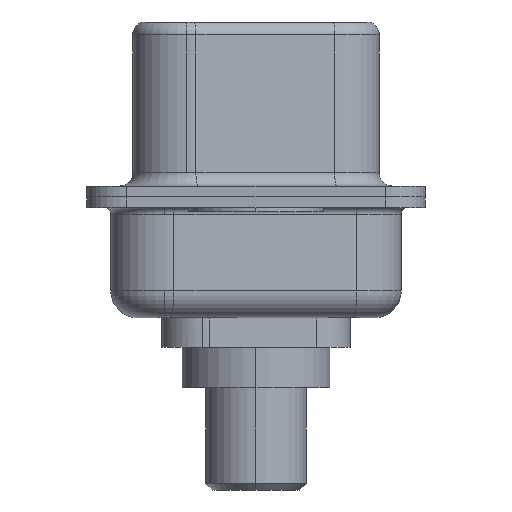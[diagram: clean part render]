
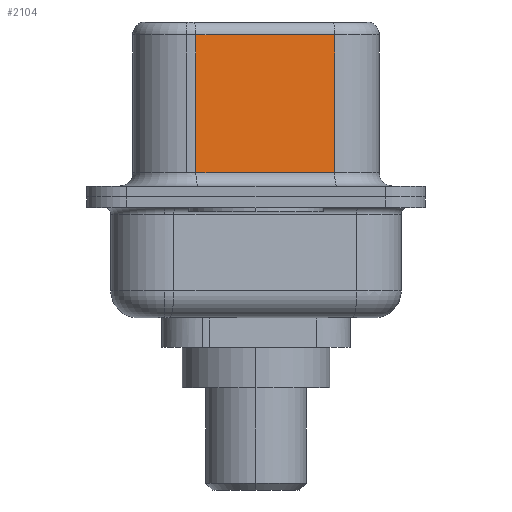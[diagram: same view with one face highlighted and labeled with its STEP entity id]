
A CAD part, left-side view. The second image highlights one B-rep face of the part: STEP entity #2104.
In plain terms, the highlighted planar face has unit normal (-0.985, -0.174, 0).
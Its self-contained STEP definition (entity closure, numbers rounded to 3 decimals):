
#248 = PLANE ( 'NONE',  #9617 ) ;
#559 = VECTOR ( 'NONE', #8483, 1000. ) ;
#745 = ORIENTED_EDGE ( 'NONE', *, *, #12222, .T. ) ;
#1006 = DIRECTION ( 'NONE',  ( -0.174, 0.985, 0. ) ) ;
#1617 = LINE ( 'NONE', #11188, #9682 ) ;
#2104 = ADVANCED_FACE ( 'NONE', ( #5008 ), #248, .F. ) ;
#2710 = VERTEX_POINT ( 'NONE', #4059 ) ;
#2716 = VECTOR ( 'NONE', #4438, 1000. ) ;
#3875 = LINE ( 'NONE', #8661, #12295 ) ;
#4059 = CARTESIAN_POINT ( 'NONE',  ( 4.565, -2.927, 0.9 ) ) ;
#4246 = EDGE_CURVE ( 'NONE', #11833, #2710, #3875, .T. ) ;
#4438 = DIRECTION ( 'NONE',  ( 0.174, -0.985, 0. ) ) ;
#4472 = CARTESIAN_POINT ( 'NONE',  ( 4.565, -2.927, 0.9 ) ) ;
#5008 = FACE_OUTER_BOUND ( 'NONE', #8089, .T. ) ;
#5394 = LINE ( 'NONE', #4472, #2716 ) ;
#6301 = ORIENTED_EDGE ( 'NONE', *, *, #11451, .T. ) ;
#6563 = CARTESIAN_POINT ( 'NONE',  ( 4.565, -2.927, 6.02 ) ) ;
#6676 = DIRECTION ( 'NONE',  ( 0.985, 0.174, 0. ) ) ;
#7121 = EDGE_CURVE ( 'NONE', #9130, #2710, #5394, .T. ) ;
#7491 = CARTESIAN_POINT ( 'NONE',  ( 3.655, 2.233, 6.02 ) ) ;
#8089 = EDGE_LOOP ( 'NONE', ( #8519, #745, #6301, #8365 ) ) ;
#8131 = DIRECTION ( 'NONE',  ( 0., 0., -1. ) ) ;
#8365 = ORIENTED_EDGE ( 'NONE', *, *, #7121, .T. ) ;
#8483 = DIRECTION ( 'NONE',  ( -0.174, 0.985, 0. ) ) ;
#8519 = ORIENTED_EDGE ( 'NONE', *, *, #4246, .F. ) ;
#8661 = CARTESIAN_POINT ( 'NONE',  ( 4.565, -2.927, 6.52 ) ) ;
#9130 = VERTEX_POINT ( 'NONE', #13201 ) ;
#9617 = AXIS2_PLACEMENT_3D ( 'NONE', #13203, #6676, #1006 ) ;
#9682 = VECTOR ( 'NONE', #8131, 1000. ) ;
#10248 = DIRECTION ( 'NONE',  ( 0., 0., -1. ) ) ;
#11133 = LINE ( 'NONE', #13647, #559 ) ;
#11170 = VERTEX_POINT ( 'NONE', #7491 ) ;
#11188 = CARTESIAN_POINT ( 'NONE',  ( 3.655, 2.233, 6.52 ) ) ;
#11451 = EDGE_CURVE ( 'NONE', #11170, #9130, #1617, .T. ) ;
#11833 = VERTEX_POINT ( 'NONE', #6563 ) ;
#12222 = EDGE_CURVE ( 'NONE', #11833, #11170, #11133, .T. ) ;
#12295 = VECTOR ( 'NONE', #10248, 1000. ) ;
#13201 = CARTESIAN_POINT ( 'NONE',  ( 3.655, 2.233, 0.9 ) ) ;
#13203 = CARTESIAN_POINT ( 'NONE',  ( 4.565, -2.927, 6.52 ) ) ;
#13647 = CARTESIAN_POINT ( 'NONE',  ( 4.565, -2.927, 6.02 ) ) ;
